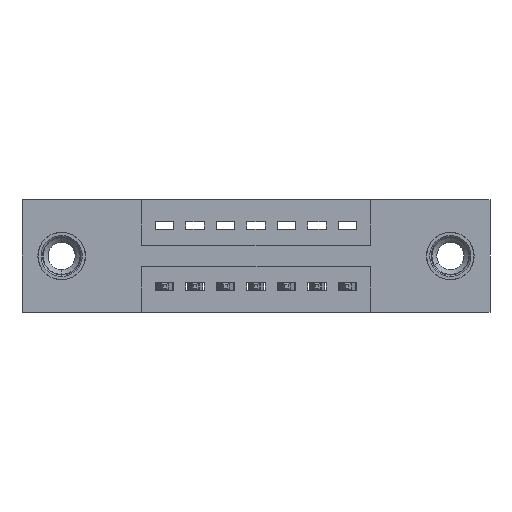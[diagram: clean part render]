
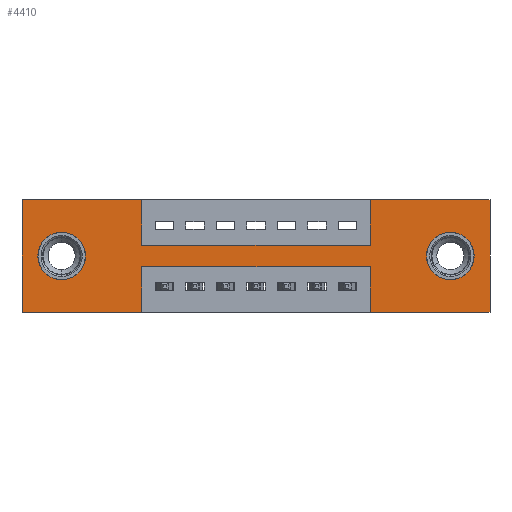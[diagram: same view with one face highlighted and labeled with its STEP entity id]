
A CAD part, front view. The second image highlights one B-rep face of the part: STEP entity #4410.
In plain terms, the highlighted planar face has unit normal (0, -1, 0).
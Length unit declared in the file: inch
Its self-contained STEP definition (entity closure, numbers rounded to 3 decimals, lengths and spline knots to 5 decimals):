
#60 = EDGE_CURVE ( 'NONE', #7542, #6378, #7135, .T. ) ;
#97 = CARTESIAN_POINT ( 'NONE',  ( 0.13, 0., -0.185 ) ) ;
#243 = CARTESIAN_POINT ( 'NONE',  ( 0.3925, 0., 0. ) ) ;
#263 = CARTESIAN_POINT ( 'NONE',  ( 0., 0., 0. ) ) ;
#286 = CARTESIAN_POINT ( 'NONE',  ( 0.3925, 0., -0.22 ) ) ;
#312 = VERTEX_POINT ( 'NONE', #476 ) ;
#328 = AXIS2_PLACEMENT_3D ( 'NONE', #6584, #8494, #8428 ) ;
#344 = VECTOR ( 'NONE', #1646, 39.37008 ) ;
#346 = FACE_BOUND ( 'NONE', #3413, .T. ) ;
#476 = CARTESIAN_POINT ( 'NONE',  ( 0.3925, 0., 0. ) ) ;
#578 = EDGE_CURVE ( 'NONE', #6378, #7542, #9525, .T. ) ;
#602 = CARTESIAN_POINT ( 'NONE',  ( 1.1425, 0., -0.15 ) ) ;
#717 = DIRECTION ( 'NONE',  ( 0., -1., 0. ) ) ;
#1115 = CARTESIAN_POINT ( 'NONE',  ( 0.13, 0., -0.107 ) ) ;
#1288 = DIRECTION ( 'NONE',  ( 0., 0., 1. ) ) ;
#1345 = EDGE_CURVE ( 'NONE', #7786, #4557, #2609, .T. ) ;
#1419 = EDGE_CURVE ( 'NONE', #7396, #4246, #1998, .T. ) ;
#1474 = VERTEX_POINT ( 'NONE', #9609 ) ;
#1481 = CARTESIAN_POINT ( 'NONE',  ( 1.535, 0., -0.37 ) ) ;
#1646 = DIRECTION ( 'NONE',  ( 1., 0., 0. ) ) ;
#1772 = CARTESIAN_POINT ( 'NONE',  ( 1.535, 0., 0. ) ) ;
#1800 = ORIENTED_EDGE ( 'NONE', *, *, #6222, .F. ) ;
#1905 = VECTOR ( 'NONE', #10550, 39.37008 ) ;
#1910 = ORIENTED_EDGE ( 'NONE', *, *, #7367, .T. ) ;
#1998 = LINE ( 'NONE', #286, #6454 ) ;
#2056 = VERTEX_POINT ( 'NONE', #5549 ) ;
#2133 = CARTESIAN_POINT ( 'NONE',  ( 1.1425, 0., -0.37 ) ) ;
#2144 = CARTESIAN_POINT ( 'NONE',  ( 1.405, 0., -0.185 ) ) ;
#2165 = VERTEX_POINT ( 'NONE', #6514 ) ;
#2198 = ORIENTED_EDGE ( 'NONE', *, *, #8337, .F. ) ;
#2267 = DIRECTION ( 'NONE',  ( -1., 0., 0. ) ) ;
#2277 = ORIENTED_EDGE ( 'NONE', *, *, #9498, .F. ) ;
#2329 = ORIENTED_EDGE ( 'NONE', *, *, #5993, .F. ) ;
#2331 = EDGE_CURVE ( 'NONE', #7192, #9680, #3474, .T. ) ;
#2345 = VECTOR ( 'NONE', #3082, 39.37008 ) ;
#2453 = VECTOR ( 'NONE', #6659, 39.37008 ) ;
#2609 = LINE ( 'NONE', #3390, #9152 ) ;
#2679 = CARTESIAN_POINT ( 'NONE',  ( 1.1425, 0., 0. ) ) ;
#2681 = DIRECTION ( 'NONE',  ( -1., 0., 0. ) ) ;
#2736 = LINE ( 'NONE', #5925, #3760 ) ;
#2766 = ORIENTED_EDGE ( 'NONE', *, *, #2331, .F. ) ;
#2902 = CARTESIAN_POINT ( 'NONE',  ( 0.3925, 0., -0.37 ) ) ;
#2955 = LINE ( 'NONE', #10919, #344 ) ;
#2996 = CARTESIAN_POINT ( 'NONE',  ( 0.13, 0., -0.263 ) ) ;
#3082 = DIRECTION ( 'NONE',  ( 0., 0., 1. ) ) ;
#3093 = DIRECTION ( 'NONE',  ( 0., 0., -1. ) ) ;
#3189 = CARTESIAN_POINT ( 'NONE',  ( 0.3925, 0., -0.37 ) ) ;
#3214 = VECTOR ( 'NONE', #1288, 39.37008 ) ;
#3390 = CARTESIAN_POINT ( 'NONE',  ( 0., 0., -0.37 ) ) ;
#3413 = EDGE_LOOP ( 'NONE', ( #1910, #5456 ) ) ;
#3474 = LINE ( 'NONE', #9134, #7473 ) ;
#3538 = DIRECTION ( 'NONE',  ( -1., 0., 0. ) ) ;
#3760 = VECTOR ( 'NONE', #9196, 39.37008 ) ;
#4246 = VERTEX_POINT ( 'NONE', #4889 ) ;
#4410 = ADVANCED_FACE ( 'NONE', ( #346, #7557, #7293 ), #8534, .T. ) ;
#4442 = VERTEX_POINT ( 'NONE', #1772 ) ;
#4473 = CIRCLE ( 'NONE', #5724, 0.078 ) ;
#4511 = ORIENTED_EDGE ( 'NONE', *, *, #4565, .F. ) ;
#4557 = VERTEX_POINT ( 'NONE', #8043 ) ;
#4565 = EDGE_CURVE ( 'NONE', #4246, #10865, #7930, .T. ) ;
#4668 = EDGE_CURVE ( 'NONE', #4442, #7786, #9084, .T. ) ;
#4702 = VECTOR ( 'NONE', #10854, 39.37008 ) ;
#4889 = CARTESIAN_POINT ( 'NONE',  ( 0.3925, 0., -0.22 ) ) ;
#4963 = CARTESIAN_POINT ( 'NONE',  ( 0., 0., -0.37 ) ) ;
#5456 = ORIENTED_EDGE ( 'NONE', *, *, #8830, .T. ) ;
#5477 = CARTESIAN_POINT ( 'NONE',  ( 1.405, 0., -0.185 ) ) ;
#5549 = CARTESIAN_POINT ( 'NONE',  ( 0.3925, 0., -0.15 ) ) ;
#5709 = AXIS2_PLACEMENT_3D ( 'NONE', #97, #8993, #8560 ) ;
#5720 = VECTOR ( 'NONE', #10421, 39.37008 ) ;
#5724 = AXIS2_PLACEMENT_3D ( 'NONE', #2144, #8209, #3093 ) ;
#5796 = CARTESIAN_POINT ( 'NONE',  ( 0., 0., 0. ) ) ;
#5810 = LINE ( 'NONE', #263, #3214 ) ;
#5856 = EDGE_LOOP ( 'NONE', ( #8592, #9626 ) ) ;
#5925 = CARTESIAN_POINT ( 'NONE',  ( 0., 0., 0. ) ) ;
#5993 = EDGE_CURVE ( 'NONE', #10865, #2165, #10296, .T. ) ;
#6222 = EDGE_CURVE ( 'NONE', #9680, #4442, #2955, .T. ) ;
#6329 = DIRECTION ( 'NONE',  ( 0., 0., -1. ) ) ;
#6378 = VERTEX_POINT ( 'NONE', #1115 ) ;
#6454 = VECTOR ( 'NONE', #3538, 39.37008 ) ;
#6477 = VERTEX_POINT ( 'NONE', #5796 ) ;
#6514 = CARTESIAN_POINT ( 'NONE',  ( 0., 0., -0.37 ) ) ;
#6573 = LINE ( 'NONE', #2133, #2345 ) ;
#6584 = CARTESIAN_POINT ( 'NONE',  ( 0.13, 0., -0.185 ) ) ;
#6659 = DIRECTION ( 'NONE',  ( 0., 0., -1. ) ) ;
#6827 = CARTESIAN_POINT ( 'NONE',  ( 1.405, 0., -0.107 ) ) ;
#7038 = ORIENTED_EDGE ( 'NONE', *, *, #7578, .F. ) ;
#7053 = DIRECTION ( 'NONE',  ( 0., 0., -1. ) ) ;
#7135 = CIRCLE ( 'NONE', #328, 0.078 ) ;
#7192 = VERTEX_POINT ( 'NONE', #602 ) ;
#7293 = FACE_OUTER_BOUND ( 'NONE', #9719, .T. ) ;
#7367 = EDGE_CURVE ( 'NONE', #8448, #1474, #11099, .T. ) ;
#7396 = VERTEX_POINT ( 'NONE', #10372 ) ;
#7473 = VECTOR ( 'NONE', #10625, 39.37008 ) ;
#7542 = VERTEX_POINT ( 'NONE', #2996 ) ;
#7557 = FACE_BOUND ( 'NONE', #5856, .T. ) ;
#7578 = EDGE_CURVE ( 'NONE', #4557, #7396, #6573, .T. ) ;
#7786 = VERTEX_POINT ( 'NONE', #1481 ) ;
#7930 = LINE ( 'NONE', #2902, #5720 ) ;
#7938 = VECTOR ( 'NONE', #2267, 39.37008 ) ;
#8043 = CARTESIAN_POINT ( 'NONE',  ( 1.1425, 0., -0.37 ) ) ;
#8142 = ORIENTED_EDGE ( 'NONE', *, *, #4668, .F. ) ;
#8187 = CARTESIAN_POINT ( 'NONE',  ( 1.535, 0., 0. ) ) ;
#8209 = DIRECTION ( 'NONE',  ( 0., 1., 0. ) ) ;
#8337 = EDGE_CURVE ( 'NONE', #2165, #6477, #5810, .T. ) ;
#8403 = ORIENTED_EDGE ( 'NONE', *, *, #1345, .F. ) ;
#8428 = DIRECTION ( 'NONE',  ( 0., 0., 1. ) ) ;
#8448 = VERTEX_POINT ( 'NONE', #6827 ) ;
#8494 = DIRECTION ( 'NONE',  ( 0., 1., 0. ) ) ;
#8530 = ORIENTED_EDGE ( 'NONE', *, *, #10429, .F. ) ;
#8534 = PLANE ( 'NONE',  #9324 ) ;
#8560 = DIRECTION ( 'NONE',  ( 0., 0., 1. ) ) ;
#8592 = ORIENTED_EDGE ( 'NONE', *, *, #578, .T. ) ;
#8830 = EDGE_CURVE ( 'NONE', #1474, #8448, #4473, .T. ) ;
#8858 = ORIENTED_EDGE ( 'NONE', *, *, #1419, .F. ) ;
#8993 = DIRECTION ( 'NONE',  ( 0., 1., 0. ) ) ;
#9084 = LINE ( 'NONE', #8187, #1905 ) ;
#9134 = CARTESIAN_POINT ( 'NONE',  ( 1.1425, 0., 0. ) ) ;
#9152 = VECTOR ( 'NONE', #2681, 39.37008 ) ;
#9196 = DIRECTION ( 'NONE',  ( 1., 0., 0. ) ) ;
#9324 = AXIS2_PLACEMENT_3D ( 'NONE', #10098, #717, #7053 ) ;
#9409 = EDGE_CURVE ( 'NONE', #312, #2056, #11050, .T. ) ;
#9498 = EDGE_CURVE ( 'NONE', #6477, #312, #2736, .T. ) ;
#9525 = CIRCLE ( 'NONE', #5709, 0.078 ) ;
#9609 = CARTESIAN_POINT ( 'NONE',  ( 1.405, 0., -0.263 ) ) ;
#9626 = ORIENTED_EDGE ( 'NONE', *, *, #60, .T. ) ;
#9680 = VERTEX_POINT ( 'NONE', #2679 ) ;
#9719 = EDGE_LOOP ( 'NONE', ( #4511, #8858, #7038, #8403, #8142, #1800, #2766, #8530, #10897, #2277, #2198, #2329 ) ) ;
#10093 = CARTESIAN_POINT ( 'NONE',  ( 0.3925, 0., -0.15 ) ) ;
#10098 = CARTESIAN_POINT ( 'NONE',  ( 0., 0., -0.37 ) ) ;
#10296 = LINE ( 'NONE', #4963, #7938 ) ;
#10372 = CARTESIAN_POINT ( 'NONE',  ( 1.1425, 0., -0.22 ) ) ;
#10421 = DIRECTION ( 'NONE',  ( 0., 0., -1. ) ) ;
#10429 = EDGE_CURVE ( 'NONE', #2056, #7192, #11146, .T. ) ;
#10550 = DIRECTION ( 'NONE',  ( 0., 0., -1. ) ) ;
#10625 = DIRECTION ( 'NONE',  ( 0., 0., 1. ) ) ;
#10854 = DIRECTION ( 'NONE',  ( 1., 0., 0. ) ) ;
#10865 = VERTEX_POINT ( 'NONE', #3189 ) ;
#10897 = ORIENTED_EDGE ( 'NONE', *, *, #9409, .F. ) ;
#10919 = CARTESIAN_POINT ( 'NONE',  ( 0., 0., 0. ) ) ;
#11028 = AXIS2_PLACEMENT_3D ( 'NONE', #5477, #11106, #6329 ) ;
#11050 = LINE ( 'NONE', #243, #2453 ) ;
#11099 = CIRCLE ( 'NONE', #11028, 0.078 ) ;
#11106 = DIRECTION ( 'NONE',  ( 0., 1., 0. ) ) ;
#11146 = LINE ( 'NONE', #10093, #4702 ) ;
